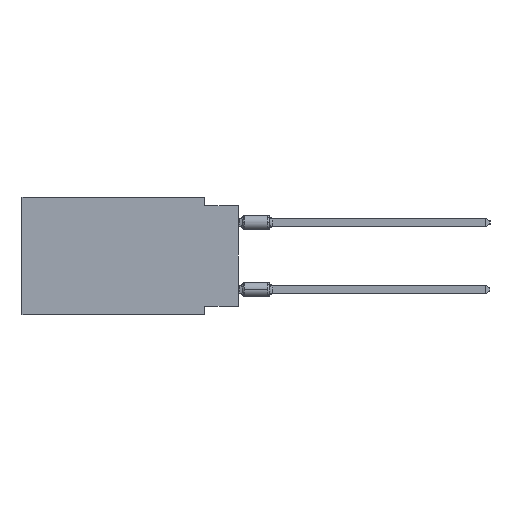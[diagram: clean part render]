
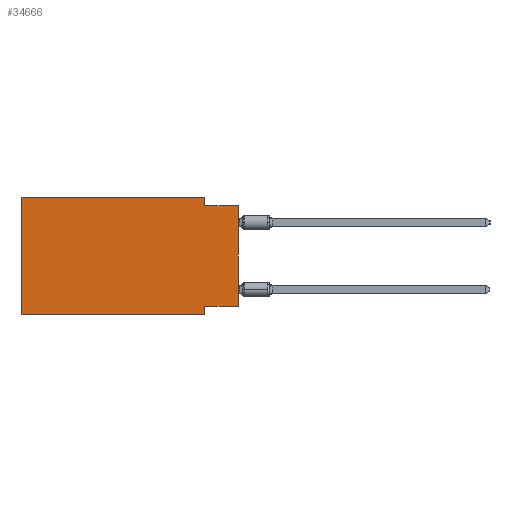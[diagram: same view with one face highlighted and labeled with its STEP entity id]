
A CAD part, left-side view. The second image highlights one B-rep face of the part: STEP entity #34666.
In plain terms, the highlighted planar face has unit normal (-1, 0, 0).
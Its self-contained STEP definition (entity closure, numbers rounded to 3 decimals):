
#133 = DIRECTION ( 'NONE',  ( 0., 0., -1. ) ) ;
#533 = CARTESIAN_POINT ( 'NONE',  ( 0., 2.54, 0. ) ) ;
#566 = VECTOR ( 'NONE', #15982, 1000. ) ;
#1349 = VECTOR ( 'NONE', #38289, 1000. ) ;
#1358 = EDGE_LOOP ( 'NONE', ( #21364, #41892, #36699, #40632, #21478, #21152, #35888, #39148 ) ) ;
#1726 = DIRECTION ( 'NONE',  ( 0., -1., 0. ) ) ;
#2376 = DIRECTION ( 'NONE',  ( 0., 1., 0. ) ) ;
#3258 = VERTEX_POINT ( 'NONE', #3927 ) ;
#3909 = CARTESIAN_POINT ( 'NONE',  ( 0., 2.54, 0. ) ) ;
#3927 = CARTESIAN_POINT ( 'NONE',  ( 0., 2.54, -8.255 ) ) ;
#4013 = VERTEX_POINT ( 'NONE', #4110 ) ;
#4110 = CARTESIAN_POINT ( 'NONE',  ( 0., 16.383, -8.89 ) ) ;
#4798 = EDGE_CURVE ( 'NONE', #26174, #34235, #35039, .T. ) ;
#5332 = CARTESIAN_POINT ( 'NONE',  ( 0., 0., 0. ) ) ;
#5868 = VERTEX_POINT ( 'NONE', #3909 ) ;
#6808 = CARTESIAN_POINT ( 'NONE',  ( 0., 2.54, -8.89 ) ) ;
#7029 = LINE ( 'NONE', #6808, #22902 ) ;
#10722 = DIRECTION ( 'NONE',  ( 0., 0., -1. ) ) ;
#13367 = CARTESIAN_POINT ( 'NONE',  ( 0., 2.54, -8.89 ) ) ;
#13539 = CARTESIAN_POINT ( 'NONE',  ( 0., 16.383, 0. ) ) ;
#15982 = DIRECTION ( 'NONE',  ( 0., 0., 1. ) ) ;
#17828 = EDGE_CURVE ( 'NONE', #22665, #5868, #41748, .T. ) ;
#18528 = VECTOR ( 'NONE', #10722, 1000. ) ;
#18558 = DIRECTION ( 'NONE',  ( 0., 0., 1. ) ) ;
#18635 = CARTESIAN_POINT ( 'NONE',  ( 0., 16.383, -8.89 ) ) ;
#19221 = DIRECTION ( 'NONE',  ( 0., -1., 0. ) ) ;
#20198 = AXIS2_PLACEMENT_3D ( 'NONE', #39832, #22903, #133 ) ;
#20892 = EDGE_CURVE ( 'NONE', #4013, #22665, #38543, .T. ) ;
#21152 = ORIENTED_EDGE ( 'NONE', *, *, #25068, .T. ) ;
#21364 = ORIENTED_EDGE ( 'NONE', *, *, #4798, .T. ) ;
#21478 = ORIENTED_EDGE ( 'NONE', *, *, #20892, .F. ) ;
#21676 = LINE ( 'NONE', #42061, #31743 ) ;
#22665 = VERTEX_POINT ( 'NONE', #13539 ) ;
#22902 = VECTOR ( 'NONE', #33271, 1000. ) ;
#22903 = DIRECTION ( 'NONE',  ( 1., 0., 0. ) ) ;
#25011 = EDGE_CURVE ( 'NONE', #26174, #3258, #21676, .T. ) ;
#25068 = EDGE_CURVE ( 'NONE', #4013, #28991, #35117, .T. ) ;
#26041 = VECTOR ( 'NONE', #18558, 1000. ) ;
#26174 = VERTEX_POINT ( 'NONE', #37965 ) ;
#28991 = VERTEX_POINT ( 'NONE', #13367 ) ;
#29341 = EDGE_CURVE ( 'NONE', #3258, #28991, #7029, .T. ) ;
#29769 = CARTESIAN_POINT ( 'NONE',  ( 0., 2.54, -0.635 ) ) ;
#30700 = EDGE_CURVE ( 'NONE', #5868, #36216, #40228, .T. ) ;
#31743 = VECTOR ( 'NONE', #2376, 1000. ) ;
#31894 = CARTESIAN_POINT ( 'NONE',  ( 0., 0., -0.635 ) ) ;
#33271 = DIRECTION ( 'NONE',  ( 0., 0., -1. ) ) ;
#33685 = LINE ( 'NONE', #40207, #41752 ) ;
#34235 = VERTEX_POINT ( 'NONE', #31894 ) ;
#34666 = ADVANCED_FACE ( 'NONE', ( #42642 ), #39393, .F. ) ;
#35039 = LINE ( 'NONE', #5332, #26041 ) ;
#35067 = CARTESIAN_POINT ( 'NONE',  ( 0., 16.383, 0. ) ) ;
#35117 = LINE ( 'NONE', #18635, #35914 ) ;
#35241 = CARTESIAN_POINT ( 'NONE',  ( 0., 16.383, 0. ) ) ;
#35888 = ORIENTED_EDGE ( 'NONE', *, *, #29341, .F. ) ;
#35914 = VECTOR ( 'NONE', #1726, 1000. ) ;
#36216 = VERTEX_POINT ( 'NONE', #29769 ) ;
#36699 = ORIENTED_EDGE ( 'NONE', *, *, #30700, .F. ) ;
#37965 = CARTESIAN_POINT ( 'NONE',  ( 0., 0., -8.255 ) ) ;
#38289 = DIRECTION ( 'NONE',  ( 0., -1., 0. ) ) ;
#38543 = LINE ( 'NONE', #35067, #566 ) ;
#39148 = ORIENTED_EDGE ( 'NONE', *, *, #25011, .F. ) ;
#39393 = PLANE ( 'NONE',  #20198 ) ;
#39832 = CARTESIAN_POINT ( 'NONE',  ( 0., 16.383, 0. ) ) ;
#40207 = CARTESIAN_POINT ( 'NONE',  ( 0., 0., -0.635 ) ) ;
#40228 = LINE ( 'NONE', #533, #18528 ) ;
#40632 = ORIENTED_EDGE ( 'NONE', *, *, #17828, .F. ) ;
#41748 = LINE ( 'NONE', #35241, #1349 ) ;
#41752 = VECTOR ( 'NONE', #19221, 1000. ) ;
#41892 = ORIENTED_EDGE ( 'NONE', *, *, #42862, .F. ) ;
#42061 = CARTESIAN_POINT ( 'NONE',  ( 0., 0., -8.255 ) ) ;
#42642 = FACE_OUTER_BOUND ( 'NONE', #1358, .T. ) ;
#42862 = EDGE_CURVE ( 'NONE', #36216, #34235, #33685, .T. ) ;
